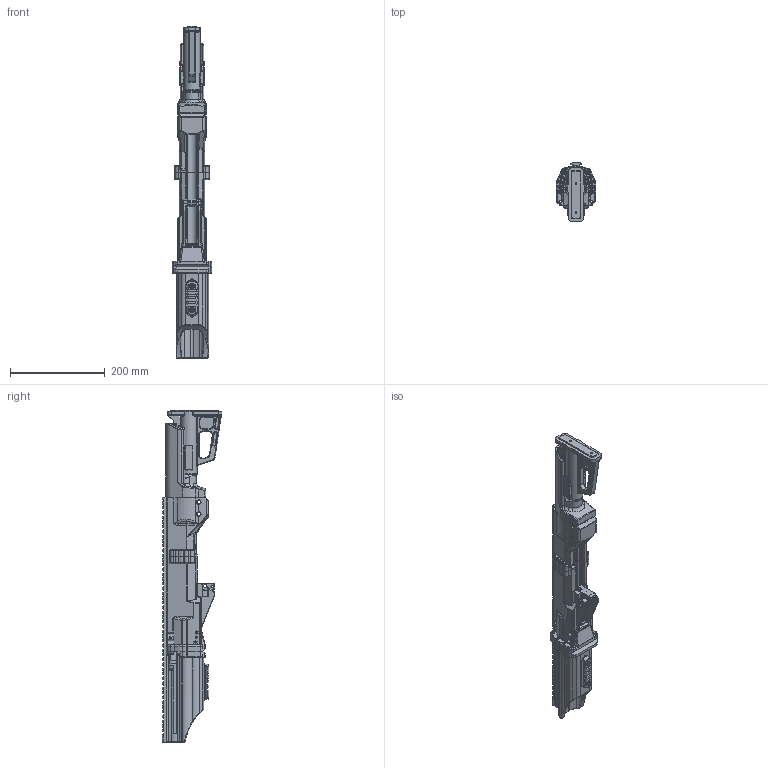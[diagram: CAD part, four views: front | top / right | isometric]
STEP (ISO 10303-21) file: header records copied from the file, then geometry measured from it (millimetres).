
FILE_DESCRIPTION(/* description */ (''),/* implementation_level */ '2;1');
FILE_NAME(/* name */ 'Amigo Grande Printed Part Assembly Rev10.stp',/* time_stamp */ '2022-03-20T13:47:45-05:00',/* author */ ('johne'),/* organization */ (''),/* preprocessor_version */ 'ST-DEVELOPER v18.1',/* originating_system */ 'Autodesk Inventor 2020',/* authorisation */ '');
FILE_SCHEMA (('AUTOMOTIVE_DESIGN { 1 0 10303 214 3 1 1 }'));
Products named in the file (8): Amigo Grande Printed Part Assembly Rev9; Handguard-Cocking Tube; Rear Receiver; Front Receiver Rev8; Barrel Mount Right Rev7; Barrel Mount Left Rev7; Foregrip Mount Pic Rail; Pho_Spuhr_V2_Assembly
Assembly tree (7 placements, depth 2):
  Amigo Grande Printed Part Assembly Rev9
    Handguard-Cocking Tube
    Rear Receiver
    Front Receiver Rev8
    Barrel Mount Right Rev7
    Barrel Mount Left Rev7
    Foregrip Mount Pic Rail
    Pho_Spuhr_V2_Assembly
Bounding box: 82.76 x 126.07 x 699.78 mm (x, y, z)
Volume: 1458840.5 mm3; surface area: 429745.8 mm2
Topology: 12 solids, 12 shells, 2836 faces, 7471 edges, 4591 vertices
Faces by surface type: plane 1002, cylinder 969, bspline 471, torus 326, sphere 48, cone 20
Full cylindrical faces by diameter (mm): 2.286 x10, 2.75 x1, 3.81 x1, 4 x40, 4.2 x2, 4.826 x2, 5 x25, 6 x1, 6.401 x1, 6.477 x2, 7 x4, 8.509 x1, 9.525 x1, 10 x2, 12.725 x1, 20.599 x1, 26.924 x1, 27.813 x1, 35.433 x1
Entity records: 104104 total; most frequent: CARTESIAN_POINT 34341, ORIENTED_EDGE 14822, DIRECTION 14377, EDGE_CURVE 7411, AXIS2_PLACEMENT_3D 5360, VERTEX_POINT 4591, LINE 3657, VECTOR 3657
